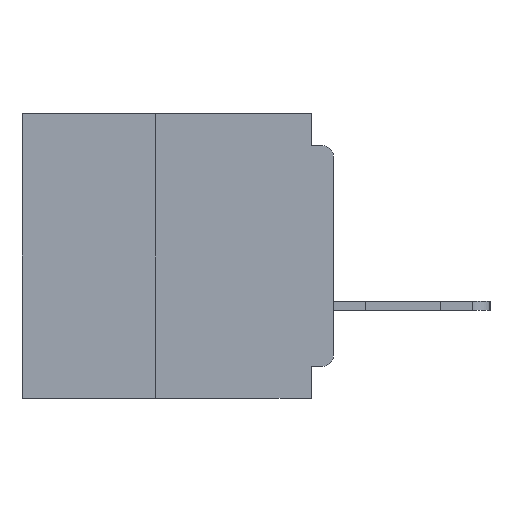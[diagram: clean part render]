
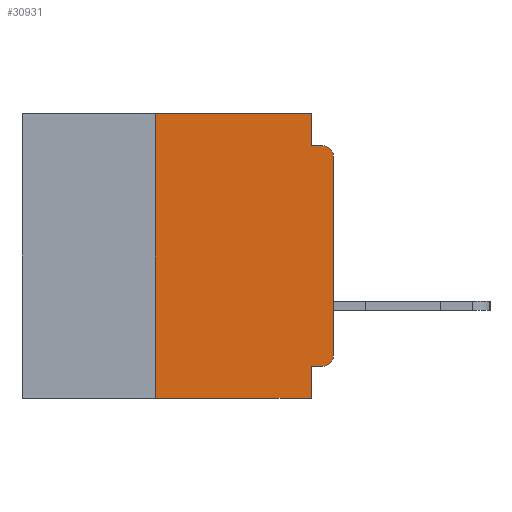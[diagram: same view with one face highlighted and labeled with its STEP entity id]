
A CAD part, left-side view. The second image highlights one B-rep face of the part: STEP entity #30931.
In plain terms, the highlighted planar face has unit normal (-1, 0, 0).
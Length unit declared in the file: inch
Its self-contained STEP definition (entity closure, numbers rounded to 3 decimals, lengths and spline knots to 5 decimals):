
#1393 = VERTEX_POINT ( 'NONE', #37857 ) ;
#2574 = CARTESIAN_POINT ( 'NONE',  ( 0., 0.031, -0.4 ) ) ;
#3085 = VECTOR ( 'NONE', #21649, 39.37008 ) ;
#3171 = LINE ( 'NONE', #3634, #28836 ) ;
#3634 = CARTESIAN_POINT ( 'NONE',  ( 0., 0., -0.045 ) ) ;
#3662 = CARTESIAN_POINT ( 'NONE',  ( 0., 0.031, -0.355 ) ) ;
#3814 = EDGE_CURVE ( 'NONE', #39580, #21708, #26613, .T. ) ;
#4163 = EDGE_CURVE ( 'NONE', #1393, #7447, #21719, .T. ) ;
#4406 = DIRECTION ( 'NONE',  ( 0., 0., -1. ) ) ;
#4419 = DIRECTION ( 'NONE',  ( -1., 0., 0. ) ) ;
#4463 = CARTESIAN_POINT ( 'NONE',  ( 0., 0.015, -0.06 ) ) ;
#4986 = CARTESIAN_POINT ( 'NONE',  ( 0., 0.25, -0.4 ) ) ;
#5121 = AXIS2_PLACEMENT_3D ( 'NONE', #27732, #17281, #13926 ) ;
#5170 = CARTESIAN_POINT ( 'NONE',  ( 0., 0.031, 0. ) ) ;
#6656 = ORIENTED_EDGE ( 'NONE', *, *, #11352, .F. ) ;
#7447 = VERTEX_POINT ( 'NONE', #5170 ) ;
#7812 = EDGE_CURVE ( 'NONE', #32248, #21708, #3171, .T. ) ;
#8021 = CARTESIAN_POINT ( 'NONE',  ( 0., 0.015, -0.34 ) ) ;
#8922 = ORIENTED_EDGE ( 'NONE', *, *, #21615, .T. ) ;
#10293 = CARTESIAN_POINT ( 'NONE',  ( 0., 0.031, -0.4 ) ) ;
#10418 = PLANE ( 'NONE',  #5121 ) ;
#11352 = EDGE_CURVE ( 'NONE', #7447, #32248, #35388, .T. ) ;
#11560 = DIRECTION ( 'NONE',  ( 0., 0., -1. ) ) ;
#11817 = VECTOR ( 'NONE', #13800, 39.37008 ) ;
#12949 = AXIS2_PLACEMENT_3D ( 'NONE', #4463, #4419, #4406 ) ;
#13800 = DIRECTION ( 'NONE',  ( 0., 0., -1. ) ) ;
#13926 = DIRECTION ( 'NONE',  ( 0., 0., -1. ) ) ;
#14885 = DIRECTION ( 'NONE',  ( 0., 0., 1. ) ) ;
#15085 = CARTESIAN_POINT ( 'NONE',  ( 0., 0., -0.34 ) ) ;
#16594 = EDGE_CURVE ( 'NONE', #41169, #32171, #31561, .T. ) ;
#16602 = CARTESIAN_POINT ( 'NONE',  ( 0., 0., -0.06 ) ) ;
#17275 = CARTESIAN_POINT ( 'NONE',  ( 0., 0.25, -0.4 ) ) ;
#17281 = DIRECTION ( 'NONE',  ( 1., 0., 0. ) ) ;
#18186 = ORIENTED_EDGE ( 'NONE', *, *, #4163, .F. ) ;
#18609 = CARTESIAN_POINT ( 'NONE',  ( 0., 0.031, 0. ) ) ;
#19339 = ORIENTED_EDGE ( 'NONE', *, *, #27201, .T. ) ;
#19563 = VECTOR ( 'NONE', #14885, 39.37008 ) ;
#19672 = CARTESIAN_POINT ( 'NONE',  ( 0., 0.015, -0.355 ) ) ;
#21571 = CARTESIAN_POINT ( 'NONE',  ( 0., 0.031, -0.045 ) ) ;
#21615 = EDGE_CURVE ( 'NONE', #41169, #28451, #24435, .T. ) ;
#21649 = DIRECTION ( 'NONE',  ( 0., -1., 0. ) ) ;
#21708 = VERTEX_POINT ( 'NONE', #40007 ) ;
#21719 = LINE ( 'NONE', #22110, #3085 ) ;
#21746 = LINE ( 'NONE', #28842, #19563 ) ;
#21886 = VERTEX_POINT ( 'NONE', #2574 ) ;
#22110 = CARTESIAN_POINT ( 'NONE',  ( 0., 0.437, 0. ) ) ;
#22254 = VECTOR ( 'NONE', #44128, 39.37008 ) ;
#22460 = DIRECTION ( 'NONE',  ( 0., 0., 1. ) ) ;
#23074 = VECTOR ( 'NONE', #22460, 39.37008 ) ;
#23824 = DIRECTION ( 'NONE',  ( 0., -1., 0. ) ) ;
#24435 = CIRCLE ( 'NONE', #24641, 0.015 ) ;
#24641 = AXIS2_PLACEMENT_3D ( 'NONE', #8021, #32443, #11560 ) ;
#26003 = VECTOR ( 'NONE', #36043, 39.37008 ) ;
#26598 = CARTESIAN_POINT ( 'NONE',  ( 0., 0., -0.355 ) ) ;
#26613 = CIRCLE ( 'NONE', #12949, 0.015 ) ;
#27201 = EDGE_CURVE ( 'NONE', #28451, #39580, #21746, .T. ) ;
#27352 = EDGE_LOOP ( 'NONE', ( #19339, #39250, #30820, #6656, #18186, #27940, #36384, #34250, #44144, #8922 ) ) ;
#27732 = CARTESIAN_POINT ( 'NONE',  ( 0., 0.437, 0. ) ) ;
#27940 = ORIENTED_EDGE ( 'NONE', *, *, #29173, .F. ) ;
#28451 = VERTEX_POINT ( 'NONE', #15085 ) ;
#28836 = VECTOR ( 'NONE', #35166, 39.37008 ) ;
#28842 = CARTESIAN_POINT ( 'NONE',  ( 0., 0., 0. ) ) ;
#29173 = EDGE_CURVE ( 'NONE', #38040, #1393, #41768, .T. ) ;
#30329 = LINE ( 'NONE', #10293, #11817 ) ;
#30704 = CARTESIAN_POINT ( 'NONE',  ( 0., 0.437, -0.4 ) ) ;
#30820 = ORIENTED_EDGE ( 'NONE', *, *, #7812, .F. ) ;
#30931 = ADVANCED_FACE ( 'NONE', ( #33955 ), #10418, .F. ) ;
#31561 = LINE ( 'NONE', #26598, #22254 ) ;
#32171 = VERTEX_POINT ( 'NONE', #3662 ) ;
#32248 = VERTEX_POINT ( 'NONE', #21571 ) ;
#32443 = DIRECTION ( 'NONE',  ( -1., 0., 0. ) ) ;
#32544 = VECTOR ( 'NONE', #23824, 39.37008 ) ;
#33955 = FACE_OUTER_BOUND ( 'NONE', #27352, .T. ) ;
#33998 = EDGE_CURVE ( 'NONE', #38040, #21886, #41910, .T. ) ;
#34054 = EDGE_CURVE ( 'NONE', #32171, #21886, #30329, .T. ) ;
#34250 = ORIENTED_EDGE ( 'NONE', *, *, #34054, .F. ) ;
#35166 = DIRECTION ( 'NONE',  ( 0., -1., 0. ) ) ;
#35388 = LINE ( 'NONE', #18609, #26003 ) ;
#36043 = DIRECTION ( 'NONE',  ( 0., 0., -1. ) ) ;
#36384 = ORIENTED_EDGE ( 'NONE', *, *, #33998, .T. ) ;
#37857 = CARTESIAN_POINT ( 'NONE',  ( 0., 0.25, 0. ) ) ;
#38040 = VERTEX_POINT ( 'NONE', #17275 ) ;
#39250 = ORIENTED_EDGE ( 'NONE', *, *, #3814, .T. ) ;
#39580 = VERTEX_POINT ( 'NONE', #16602 ) ;
#40007 = CARTESIAN_POINT ( 'NONE',  ( 0., 0.015, -0.045 ) ) ;
#41169 = VERTEX_POINT ( 'NONE', #19672 ) ;
#41768 = LINE ( 'NONE', #4986, #23074 ) ;
#41910 = LINE ( 'NONE', #30704, #32544 ) ;
#44128 = DIRECTION ( 'NONE',  ( 0., 1., 0. ) ) ;
#44144 = ORIENTED_EDGE ( 'NONE', *, *, #16594, .F. ) ;
